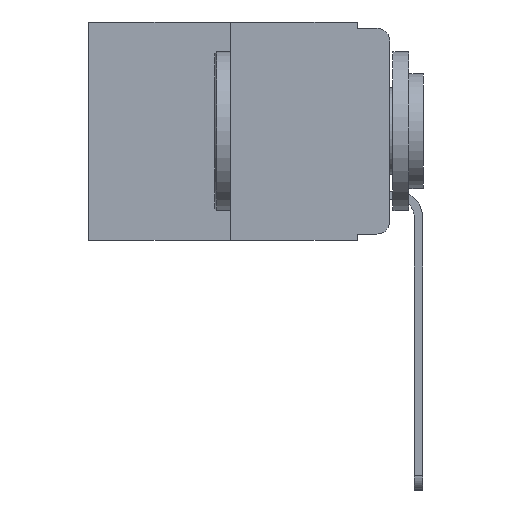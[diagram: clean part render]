
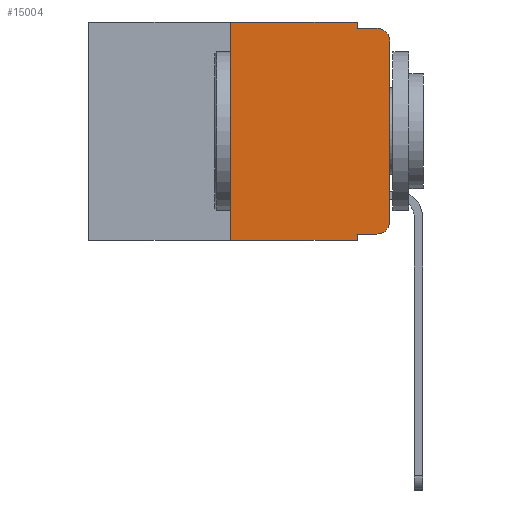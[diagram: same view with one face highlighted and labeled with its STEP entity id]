
A CAD part, left-side view. The second image highlights one B-rep face of the part: STEP entity #15004.
In plain terms, the highlighted planar face has unit normal (-1, 0, 0).
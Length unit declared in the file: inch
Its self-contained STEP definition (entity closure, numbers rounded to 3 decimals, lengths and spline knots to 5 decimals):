
#225 = VERTEX_POINT ( 'NONE', #17040 ) ;
#236 = AXIS2_PLACEMENT_3D ( 'NONE', #9246, #4137, #17771 ) ;
#248 = CARTESIAN_POINT ( 'NONE',  ( 0., 0.25, 0. ) ) ;
#1054 = ORIENTED_EDGE ( 'NONE', *, *, #8276, .T. ) ;
#1802 = VERTEX_POINT ( 'NONE', #11734 ) ;
#1851 = CARTESIAN_POINT ( 'NONE',  ( 0., 0.25, 0. ) ) ;
#2413 = EDGE_CURVE ( 'NONE', #20623, #12958, #5224, .T. ) ;
#3234 = VECTOR ( 'NONE', #17139, 39.37008 ) ;
#3676 = CARTESIAN_POINT ( 'NONE',  ( 0., 0.051, -0.01 ) ) ;
#3795 = ORIENTED_EDGE ( 'NONE', *, *, #2413, .F. ) ;
#3828 = ORIENTED_EDGE ( 'NONE', *, *, #12232, .F. ) ;
#4007 = VECTOR ( 'NONE', #10456, 39.37008 ) ;
#4137 = DIRECTION ( 'NONE',  ( 1., 0., 0. ) ) ;
#4420 = DIRECTION ( 'NONE',  ( 0., -1., 0. ) ) ;
#4465 = EDGE_CURVE ( 'NONE', #19549, #12958, #20649, .T. ) ;
#4930 = VERTEX_POINT ( 'NONE', #17820 ) ;
#4939 = DIRECTION ( 'NONE',  ( 0., 0., -1. ) ) ;
#5224 = LINE ( 'NONE', #19963, #9153 ) ;
#5564 = AXIS2_PLACEMENT_3D ( 'NONE', #21689, #14939, #4939 ) ;
#5788 = DIRECTION ( 'NONE',  ( -1., 0., 0. ) ) ;
#5848 = LINE ( 'NONE', #11824, #3234 ) ;
#6948 = EDGE_CURVE ( 'NONE', #1802, #14503, #10853, .T. ) ;
#6971 = ORIENTED_EDGE ( 'NONE', *, *, #16888, .F. ) ;
#6992 = CARTESIAN_POINT ( 'NONE',  ( 0., 0.25, -0.343 ) ) ;
#7509 = DIRECTION ( 'NONE',  ( 0., 0., -1. ) ) ;
#8188 = CIRCLE ( 'NONE', #5564, 0.02 ) ;
#8276 = EDGE_CURVE ( 'NONE', #225, #1802, #9515, .T. ) ;
#9153 = VECTOR ( 'NONE', #9652, 39.37008 ) ;
#9233 = ORIENTED_EDGE ( 'NONE', *, *, #21093, .F. ) ;
#9246 = CARTESIAN_POINT ( 'NONE',  ( 0., 0.473, 0. ) ) ;
#9495 = CARTESIAN_POINT ( 'NONE',  ( 0., 0.02, -0.01 ) ) ;
#9515 = LINE ( 'NONE', #12073, #4007 ) ;
#9584 = LINE ( 'NONE', #21288, #9859 ) ;
#9652 = DIRECTION ( 'NONE',  ( 0., 0., -1. ) ) ;
#9859 = VECTOR ( 'NONE', #21214, 39.37008 ) ;
#10076 = VECTOR ( 'NONE', #10370, 39.37008 ) ;
#10370 = DIRECTION ( 'NONE',  ( 0., 0., 1. ) ) ;
#10456 = DIRECTION ( 'NONE',  ( 0., 0., 1. ) ) ;
#10786 = AXIS2_PLACEMENT_3D ( 'NONE', #15880, #5788, #7509 ) ;
#10853 = CIRCLE ( 'NONE', #10786, 0.02 ) ;
#11734 = CARTESIAN_POINT ( 'NONE',  ( 0., 0., -0.03 ) ) ;
#11776 = CARTESIAN_POINT ( 'NONE',  ( 0., 0.051, -0.333 ) ) ;
#11824 = CARTESIAN_POINT ( 'NONE',  ( 0., 0.051, -0.333 ) ) ;
#12073 = CARTESIAN_POINT ( 'NONE',  ( 0., 0., 0. ) ) ;
#12092 = DIRECTION ( 'NONE',  ( 0., -1., 0. ) ) ;
#12232 = EDGE_CURVE ( 'NONE', #21438, #4930, #9584, .T. ) ;
#12722 = VECTOR ( 'NONE', #12092, 39.37008 ) ;
#12846 = ORIENTED_EDGE ( 'NONE', *, *, #4465, .T. ) ;
#12879 = EDGE_CURVE ( 'NONE', #19549, #18848, #14576, .T. ) ;
#12958 = VERTEX_POINT ( 'NONE', #20898 ) ;
#13011 = CARTESIAN_POINT ( 'NONE',  ( 0., 0.473, -0.343 ) ) ;
#13319 = DIRECTION ( 'NONE',  ( 0., -1., 0. ) ) ;
#13349 = EDGE_CURVE ( 'NONE', #16720, #225, #8188, .T. ) ;
#13890 = CARTESIAN_POINT ( 'NONE',  ( 0., 0.051, 0. ) ) ;
#14029 = LINE ( 'NONE', #3676, #12722 ) ;
#14503 = VERTEX_POINT ( 'NONE', #9495 ) ;
#14576 = LINE ( 'NONE', #248, #10076 ) ;
#14939 = DIRECTION ( 'NONE',  ( -1., 0., 0. ) ) ;
#15004 = ADVANCED_FACE ( 'NONE', ( #20994 ), #17493, .F. ) ;
#15880 = CARTESIAN_POINT ( 'NONE',  ( 0., 0.02, -0.03 ) ) ;
#16506 = ORIENTED_EDGE ( 'NONE', *, *, #13349, .T. ) ;
#16720 = VERTEX_POINT ( 'NONE', #20142 ) ;
#16888 = EDGE_CURVE ( 'NONE', #4930, #14503, #14029, .T. ) ;
#17040 = CARTESIAN_POINT ( 'NONE',  ( 0., 0., -0.313 ) ) ;
#17139 = DIRECTION ( 'NONE',  ( 0., -1., 0. ) ) ;
#17168 = ORIENTED_EDGE ( 'NONE', *, *, #18123, .T. ) ;
#17493 = PLANE ( 'NONE',  #236 ) ;
#17771 = DIRECTION ( 'NONE',  ( 0., 0., -1. ) ) ;
#17820 = CARTESIAN_POINT ( 'NONE',  ( 0., 0.051, -0.01 ) ) ;
#18123 = EDGE_CURVE ( 'NONE', #20623, #16720, #5848, .T. ) ;
#18523 = CARTESIAN_POINT ( 'NONE',  ( 0., 0.473, 0. ) ) ;
#18848 = VERTEX_POINT ( 'NONE', #1851 ) ;
#19033 = EDGE_LOOP ( 'NONE', ( #1054, #19655, #6971, #3828, #9233, #19787, #12846, #3795, #17168, #16506 ) ) ;
#19549 = VERTEX_POINT ( 'NONE', #6992 ) ;
#19586 = VECTOR ( 'NONE', #4420, 39.37008 ) ;
#19655 = ORIENTED_EDGE ( 'NONE', *, *, #6948, .T. ) ;
#19787 = ORIENTED_EDGE ( 'NONE', *, *, #12879, .F. ) ;
#19963 = CARTESIAN_POINT ( 'NONE',  ( 0., 0.051, 0. ) ) ;
#20142 = CARTESIAN_POINT ( 'NONE',  ( 0., 0.02, -0.333 ) ) ;
#20623 = VERTEX_POINT ( 'NONE', #11776 ) ;
#20649 = LINE ( 'NONE', #13011, #19586 ) ;
#20708 = LINE ( 'NONE', #18523, #21234 ) ;
#20898 = CARTESIAN_POINT ( 'NONE',  ( 0., 0.051, -0.343 ) ) ;
#20994 = FACE_OUTER_BOUND ( 'NONE', #19033, .T. ) ;
#21093 = EDGE_CURVE ( 'NONE', #18848, #21438, #20708, .T. ) ;
#21214 = DIRECTION ( 'NONE',  ( 0., 0., -1. ) ) ;
#21234 = VECTOR ( 'NONE', #13319, 39.37008 ) ;
#21288 = CARTESIAN_POINT ( 'NONE',  ( 0., 0.051, 0. ) ) ;
#21438 = VERTEX_POINT ( 'NONE', #13890 ) ;
#21689 = CARTESIAN_POINT ( 'NONE',  ( 0., 0.02, -0.313 ) ) ;
